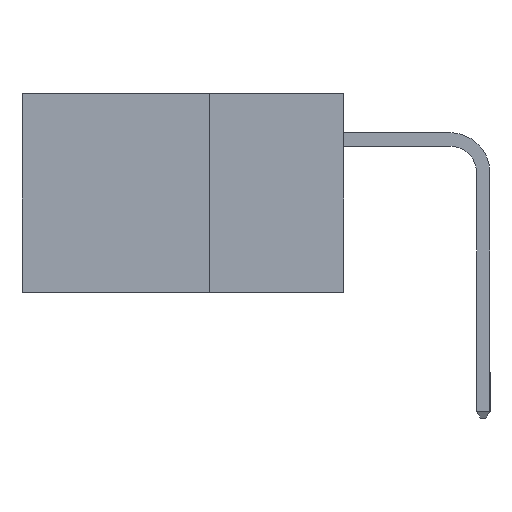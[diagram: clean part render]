
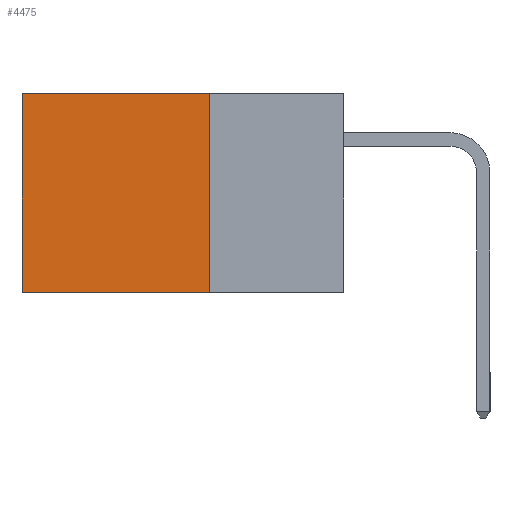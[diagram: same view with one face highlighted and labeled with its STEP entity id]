
A CAD part, left-side view. The second image highlights one B-rep face of the part: STEP entity #4475.
In plain terms, the highlighted planar face has unit normal (-1, 0, 0).
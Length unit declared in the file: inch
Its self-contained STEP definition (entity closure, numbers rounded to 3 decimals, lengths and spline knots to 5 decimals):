
#138 = DIRECTION ( 'NONE',  ( 0., 0., -1. ) ) ;
#377 = CARTESIAN_POINT ( 'NONE',  ( 0.2615, 0.6, -0.37 ) ) ;
#669 = VECTOR ( 'NONE', #7482, 39.37008 ) ;
#1149 = LINE ( 'NONE', #10393, #6331 ) ;
#1203 = CARTESIAN_POINT ( 'NONE',  ( 0.2615, 0.25, -0.37 ) ) ;
#2092 = DIRECTION ( 'NONE',  ( 1., 0., 0. ) ) ;
#2119 = CARTESIAN_POINT ( 'NONE',  ( 0.2615, 0.6, -0.37 ) ) ;
#3367 = PLANE ( 'NONE',  #6950 ) ;
#4428 = EDGE_CURVE ( 'NONE', #8652, #14780, #8497, .T. ) ;
#4442 = VERTEX_POINT ( 'NONE', #4911 ) ;
#4475 = ADVANCED_FACE ( 'NONE', ( #4649 ), #3367, .F. ) ;
#4649 = FACE_OUTER_BOUND ( 'NONE', #5867, .T. ) ;
#4837 = CARTESIAN_POINT ( 'NONE',  ( 0.2615, 0.25, 0. ) ) ;
#4911 = CARTESIAN_POINT ( 'NONE',  ( 0.2615, 0.25, -0.37 ) ) ;
#5136 = DIRECTION ( 'NONE',  ( 0., 1., 0. ) ) ;
#5158 = ORIENTED_EDGE ( 'NONE', *, *, #12521, .T. ) ;
#5532 = ORIENTED_EDGE ( 'NONE', *, *, #16800, .F. ) ;
#5867 = EDGE_LOOP ( 'NONE', ( #5158, #5532, #7442, #8896 ) ) ;
#6019 = CARTESIAN_POINT ( 'NONE',  ( 0.2615, 0.25, 0. ) ) ;
#6331 = VECTOR ( 'NONE', #138, 39.37008 ) ;
#6950 = AXIS2_PLACEMENT_3D ( 'NONE', #8586, #2092, #7302 ) ;
#7302 = DIRECTION ( 'NONE',  ( 0., 0., -1. ) ) ;
#7442 = ORIENTED_EDGE ( 'NONE', *, *, #10584, .F. ) ;
#7482 = DIRECTION ( 'NONE',  ( 0., 1., 0. ) ) ;
#8497 = LINE ( 'NONE', #6019, #669 ) ;
#8586 = CARTESIAN_POINT ( 'NONE',  ( 0.2615, 0.25, -0.37 ) ) ;
#8652 = VERTEX_POINT ( 'NONE', #4837 ) ;
#8790 = VECTOR ( 'NONE', #10852, 39.37008 ) ;
#8896 = ORIENTED_EDGE ( 'NONE', *, *, #4428, .T. ) ;
#9017 = CARTESIAN_POINT ( 'NONE',  ( 0.2615, 0.6, 0. ) ) ;
#9574 = VERTEX_POINT ( 'NONE', #377 ) ;
#10393 = CARTESIAN_POINT ( 'NONE',  ( 0.2615, 0.25, -0.37 ) ) ;
#10584 = EDGE_CURVE ( 'NONE', #8652, #4442, #1149, .T. ) ;
#10852 = DIRECTION ( 'NONE',  ( 0., 0., -1. ) ) ;
#12521 = EDGE_CURVE ( 'NONE', #14780, #9574, #13550, .T. ) ;
#13152 = VECTOR ( 'NONE', #5136, 39.37008 ) ;
#13550 = LINE ( 'NONE', #2119, #8790 ) ;
#14780 = VERTEX_POINT ( 'NONE', #9017 ) ;
#16800 = EDGE_CURVE ( 'NONE', #4442, #9574, #16802, .T. ) ;
#16802 = LINE ( 'NONE', #1203, #13152 ) ;
